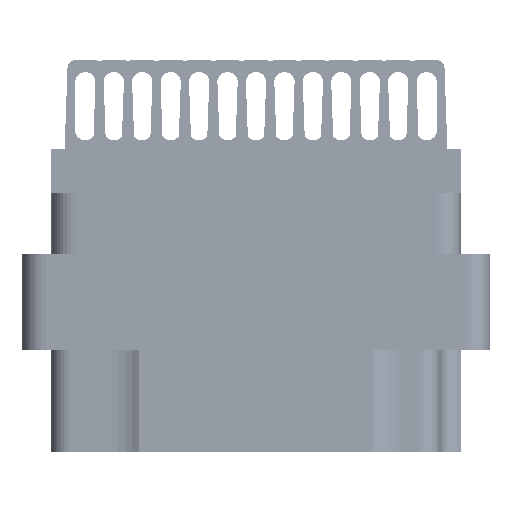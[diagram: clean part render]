
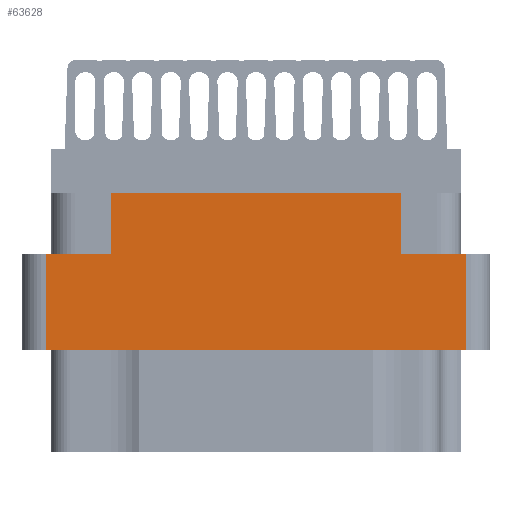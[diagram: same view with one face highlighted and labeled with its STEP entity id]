
A CAD part, left-side view. The second image highlights one B-rep face of the part: STEP entity #63628.
In plain terms, the highlighted planar face has unit normal (-1, 0, 0).
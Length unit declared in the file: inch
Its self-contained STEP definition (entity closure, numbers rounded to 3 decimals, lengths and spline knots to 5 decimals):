
#2511 = EDGE_CURVE ( 'NONE', #49341, #6498, #68248, .T. ) ;
#4772 = ORIENTED_EDGE ( 'NONE', *, *, #28150, .F. ) ;
#6498 = VERTEX_POINT ( 'NONE', #63178 ) ;
#6542 = CARTESIAN_POINT ( 'NONE',  ( -1.359, -0.617, -0.798 ) ) ;
#9130 = VECTOR ( 'NONE', #40154, 39.37008 ) ;
#10115 = ORIENTED_EDGE ( 'NONE', *, *, #2511, .T. ) ;
#10704 = VECTOR ( 'NONE', #39232, 39.37008 ) ;
#12520 = PLANE ( 'NONE',  #19855 ) ;
#12583 = LINE ( 'NONE', #24379, #9130 ) ;
#13662 = CARTESIAN_POINT ( 'NONE',  ( -1.359, -0.555, -0.529 ) ) ;
#14011 = ORIENTED_EDGE ( 'NONE', *, *, #56707, .T. ) ;
#14522 = VECTOR ( 'NONE', #15735, 39.37008 ) ;
#14841 = VECTOR ( 'NONE', #16787, 39.37008 ) ;
#15735 = DIRECTION ( 'NONE',  ( 0., -1., 0. ) ) ;
#15848 = CARTESIAN_POINT ( 'NONE',  ( -1.359, -0.555, -0.798 ) ) ;
#16787 = DIRECTION ( 'NONE',  ( 0., -1., 0. ) ) ;
#17042 = CARTESIAN_POINT ( 'NONE',  ( -1.359, 0.3825, -0.277 ) ) ;
#19253 = VERTEX_POINT ( 'NONE', #65334 ) ;
#19855 = AXIS2_PLACEMENT_3D ( 'NONE', #6542, #61186, #23245 ) ;
#20919 = CARTESIAN_POINT ( 'NONE',  ( -1.359, -0.3825, -0.277 ) ) ;
#21536 = VERTEX_POINT ( 'NONE', #70719 ) ;
#21943 = LINE ( 'NONE', #63499, #58658 ) ;
#23245 = DIRECTION ( 'NONE',  ( 0., 0., 1. ) ) ;
#23378 = VECTOR ( 'NONE', #43945, 39.37008 ) ;
#24082 = VECTOR ( 'NONE', #64103, 39.37008 ) ;
#24379 = CARTESIAN_POINT ( 'NONE',  ( -1.359, 0.3825, -0.277 ) ) ;
#25201 = LINE ( 'NONE', #44515, #10704 ) ;
#26340 = ORIENTED_EDGE ( 'NONE', *, *, #52232, .F. ) ;
#27525 = LINE ( 'NONE', #20919, #24082 ) ;
#28150 = EDGE_CURVE ( 'NONE', #44692, #60800, #66848, .T. ) ;
#28410 = CARTESIAN_POINT ( 'NONE',  ( -1.359, 0.3825, -0.117 ) ) ;
#33345 = VECTOR ( 'NONE', #37320, 39.37008 ) ;
#33805 = ORIENTED_EDGE ( 'NONE', *, *, #62757, .T. ) ;
#36088 = ORIENTED_EDGE ( 'NONE', *, *, #49441, .F. ) ;
#36890 = ORIENTED_EDGE ( 'NONE', *, *, #41957, .F. ) ;
#37320 = DIRECTION ( 'NONE',  ( 0., 0., 1. ) ) ;
#37547 = VERTEX_POINT ( 'NONE', #41387 ) ;
#39232 = DIRECTION ( 'NONE',  ( 0., 0., -1. ) ) ;
#40154 = DIRECTION ( 'NONE',  ( 0., 0., 1. ) ) ;
#41387 = CARTESIAN_POINT ( 'NONE',  ( -1.359, -0.3825, -0.117 ) ) ;
#41957 = EDGE_CURVE ( 'NONE', #62338, #37547, #58063, .T. ) ;
#43945 = DIRECTION ( 'NONE',  ( 0., -1., 0. ) ) ;
#44515 = CARTESIAN_POINT ( 'NONE',  ( -1.359, 0.555, -0.798 ) ) ;
#44692 = VERTEX_POINT ( 'NONE', #55919 ) ;
#45355 = FACE_OUTER_BOUND ( 'NONE', #57629, .T. ) ;
#48634 = CARTESIAN_POINT ( 'NONE',  ( -1.359, 0.617, -0.117 ) ) ;
#49341 = VERTEX_POINT ( 'NONE', #13662 ) ;
#49441 = EDGE_CURVE ( 'NONE', #60800, #62338, #12583, .T. ) ;
#49488 = EDGE_CURVE ( 'NONE', #49341, #19253, #21943, .T. ) ;
#52232 = EDGE_CURVE ( 'NONE', #21536, #6498, #70241, .T. ) ;
#55919 = CARTESIAN_POINT ( 'NONE',  ( -1.359, 0.555, -0.277 ) ) ;
#56707 = EDGE_CURVE ( 'NONE', #44692, #19253, #25201, .T. ) ;
#57629 = EDGE_LOOP ( 'NONE', ( #4772, #14011, #61655, #10115, #26340, #33805, #36890, #36088 ) ) ;
#58063 = LINE ( 'NONE', #48634, #14522 ) ;
#58658 = VECTOR ( 'NONE', #69189, 39.37008 ) ;
#60800 = VERTEX_POINT ( 'NONE', #17042 ) ;
#61186 = DIRECTION ( 'NONE',  ( -1., 0., 0. ) ) ;
#61655 = ORIENTED_EDGE ( 'NONE', *, *, #49488, .F. ) ;
#62338 = VERTEX_POINT ( 'NONE', #28410 ) ;
#62757 = EDGE_CURVE ( 'NONE', #21536, #37547, #27525, .T. ) ;
#63178 = CARTESIAN_POINT ( 'NONE',  ( -1.359, -0.555, -0.277 ) ) ;
#63499 = CARTESIAN_POINT ( 'NONE',  ( -1.359, 0., -0.529 ) ) ;
#63628 = ADVANCED_FACE ( 'NONE', ( #45355 ), #12520, .T. ) ;
#64103 = DIRECTION ( 'NONE',  ( 0., 0., 1. ) ) ;
#65334 = CARTESIAN_POINT ( 'NONE',  ( -1.359, 0.555, -0.529 ) ) ;
#65582 = CARTESIAN_POINT ( 'NONE',  ( -1.359, 0., -0.277 ) ) ;
#66848 = LINE ( 'NONE', #65582, #23378 ) ;
#67435 = CARTESIAN_POINT ( 'NONE',  ( -1.359, 0., -0.277 ) ) ;
#68248 = LINE ( 'NONE', #15848, #33345 ) ;
#69189 = DIRECTION ( 'NONE',  ( 0., 1., 0. ) ) ;
#70241 = LINE ( 'NONE', #67435, #14841 ) ;
#70719 = CARTESIAN_POINT ( 'NONE',  ( -1.359, -0.3825, -0.277 ) ) ;
